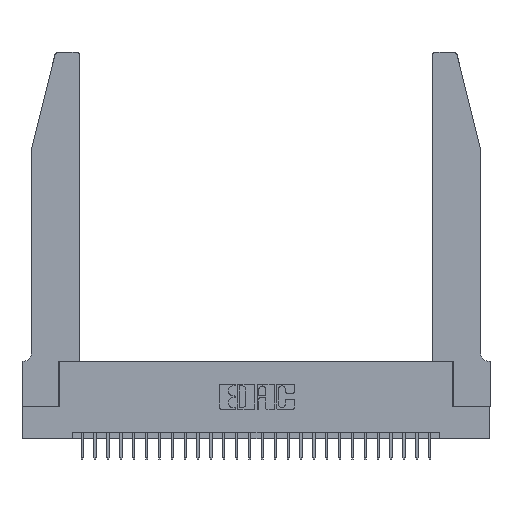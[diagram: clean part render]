
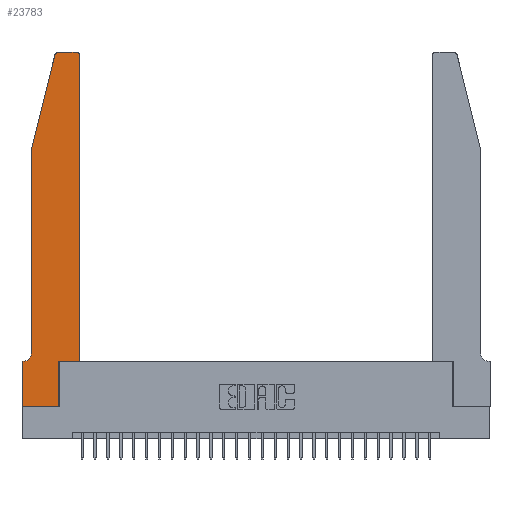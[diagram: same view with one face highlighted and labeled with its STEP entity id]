
A CAD part, top view. The second image highlights one B-rep face of the part: STEP entity #23783.
In plain terms, the highlighted planar face has unit normal (0, 0, 1).
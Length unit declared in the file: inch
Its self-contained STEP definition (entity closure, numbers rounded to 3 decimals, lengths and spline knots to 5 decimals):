
#187 = VERTEX_POINT ( 'NONE', #13765 ) ;
#409 = CARTESIAN_POINT ( 'NONE',  ( 0., 0., 0.37 ) ) ;
#474 = EDGE_LOOP ( 'NONE', ( #20091, #7254, #11517, #779, #2301, #14480, #12232, #7936, #6198, #28641, #19624, #24292 ) ) ;
#686 = AXIS2_PLACEMENT_3D ( 'NONE', #15063, #15173, #28624 ) ;
#774 = CARTESIAN_POINT ( 'NONE',  ( 0.2865, 0.35, 0.37 ) ) ;
#779 = ORIENTED_EDGE ( 'NONE', *, *, #18143, .T. ) ;
#855 = VERTEX_POINT ( 'NONE', #4358 ) ;
#983 = CARTESIAN_POINT ( 'NONE',  ( 0.0755, 2., 0.37 ) ) ;
#1223 = CARTESIAN_POINT ( 'NONE',  ( 0., 0.35, 0.37 ) ) ;
#1529 = AXIS2_PLACEMENT_3D ( 'NONE', #3961, #12609, #5810 ) ;
#2301 = ORIENTED_EDGE ( 'NONE', *, *, #15092, .T. ) ;
#3167 = VECTOR ( 'NONE', #26684, 39.37008 ) ;
#3686 = EDGE_CURVE ( 'NONE', #8865, #9156, #10705, .T. ) ;
#3943 = VECTOR ( 'NONE', #11604, 39.37008 ) ;
#3961 = CARTESIAN_POINT ( 'NONE',  ( 0.284, 2.72, 0.37 ) ) ;
#4107 = CARTESIAN_POINT ( 'NONE',  ( 0.4505, 0.35, 0.37 ) ) ;
#4358 = CARTESIAN_POINT ( 'NONE',  ( 0.4505, 2.72, 0.37 ) ) ;
#4560 = LINE ( 'NONE', #409, #3167 ) ;
#4834 = VECTOR ( 'NONE', #26246, 39.37008 ) ;
#5576 = DIRECTION ( 'NONE',  ( -0.239, -0.971, 0. ) ) ;
#5810 = DIRECTION ( 'NONE',  ( 1., 0., 0. ) ) ;
#6086 = DIRECTION ( 'NONE',  ( 1., 0., 0. ) ) ;
#6198 = ORIENTED_EDGE ( 'NONE', *, *, #3686, .T. ) ;
#6269 = LINE ( 'NONE', #23879, #4834 ) ;
#7254 = ORIENTED_EDGE ( 'NONE', *, *, #18571, .T. ) ;
#7544 = VERTEX_POINT ( 'NONE', #20810 ) ;
#7936 = ORIENTED_EDGE ( 'NONE', *, *, #14572, .T. ) ;
#7996 = PLANE ( 'NONE',  #16901 ) ;
#8092 = CIRCLE ( 'NONE', #1529, 0.03 ) ;
#8218 = DIRECTION ( 'NONE',  ( 0., 0., 1. ) ) ;
#8241 = CARTESIAN_POINT ( 'NONE',  ( 0.25487, 2.72718, 0.37 ) ) ;
#8254 = CARTESIAN_POINT ( 'NONE',  ( 0.284, 2.75, 0.37 ) ) ;
#8370 = CARTESIAN_POINT ( 'NONE',  ( 0.0755, 0.35, 0.37 ) ) ;
#8865 = VERTEX_POINT ( 'NONE', #10426 ) ;
#9140 = VECTOR ( 'NONE', #16576, 39.37008 ) ;
#9156 = VERTEX_POINT ( 'NONE', #10297 ) ;
#9300 = EDGE_CURVE ( 'NONE', #9156, #7544, #21344, .T. ) ;
#9340 = EDGE_CURVE ( 'NONE', #7544, #855, #20635, .T. ) ;
#9704 = DIRECTION ( 'NONE',  ( 0., 1., 0. ) ) ;
#9758 = DIRECTION ( 'NONE',  ( 1., 0., 0. ) ) ;
#9860 = VERTEX_POINT ( 'NONE', #14609 ) ;
#9937 = VECTOR ( 'NONE', #5576, 39.37008 ) ;
#10177 = DIRECTION ( 'NONE',  ( 0., 1., 0. ) ) ;
#10297 = CARTESIAN_POINT ( 'NONE',  ( 0.2865, 0.35, 0.37 ) ) ;
#10426 = CARTESIAN_POINT ( 'NONE',  ( 0.2865, 0., 0.37 ) ) ;
#10520 = DIRECTION ( 'NONE',  ( -1., 0., 0. ) ) ;
#10705 = LINE ( 'NONE', #774, #11374 ) ;
#10713 = VERTEX_POINT ( 'NONE', #22737 ) ;
#11374 = VECTOR ( 'NONE', #9704, 39.37008 ) ;
#11517 = ORIENTED_EDGE ( 'NONE', *, *, #16825, .T. ) ;
#11604 = DIRECTION ( 'NONE',  ( -1., 0., 0. ) ) ;
#12087 = VERTEX_POINT ( 'NONE', #12546 ) ;
#12232 = ORIENTED_EDGE ( 'NONE', *, *, #13995, .T. ) ;
#12546 = CARTESIAN_POINT ( 'NONE',  ( 0., 0.35, 0.37 ) ) ;
#12609 = DIRECTION ( 'NONE',  ( 0., 0., 1. ) ) ;
#13446 = FACE_OUTER_BOUND ( 'NONE', #474, .T. ) ;
#13765 = CARTESIAN_POINT ( 'NONE',  ( 0.4205, 2.75, 0.37 ) ) ;
#13995 = EDGE_CURVE ( 'NONE', #12087, #9860, #4560, .T. ) ;
#14399 = VERTEX_POINT ( 'NONE', #26976 ) ;
#14480 = ORIENTED_EDGE ( 'NONE', *, *, #16357, .T. ) ;
#14572 = EDGE_CURVE ( 'NONE', #9860, #8865, #6269, .T. ) ;
#14609 = CARTESIAN_POINT ( 'NONE',  ( 0., 0., 0.37 ) ) ;
#14823 = EDGE_CURVE ( 'NONE', #855, #187, #21125, .T. ) ;
#14831 = LINE ( 'NONE', #8370, #26615 ) ;
#14850 = CARTESIAN_POINT ( 'NONE',  ( 0.2605, 2.75, 0.37 ) ) ;
#15063 = CARTESIAN_POINT ( 'NONE',  ( 0.0055, 0.42, 0.37 ) ) ;
#15092 = EDGE_CURVE ( 'NONE', #17347, #14399, #21803, .T. ) ;
#15173 = DIRECTION ( 'NONE',  ( 0., 0., -1. ) ) ;
#15710 = LINE ( 'NONE', #14850, #3943 ) ;
#16357 = EDGE_CURVE ( 'NONE', #14399, #12087, #14831, .T. ) ;
#16576 = DIRECTION ( 'NONE',  ( 0., -1., 0. ) ) ;
#16825 = EDGE_CURVE ( 'NONE', #28004, #10713, #20994, .T. ) ;
#16901 = AXIS2_PLACEMENT_3D ( 'NONE', #1223, #18838, #9758 ) ;
#16982 = CARTESIAN_POINT ( 'NONE',  ( 0.4505, 0.35, 0.37 ) ) ;
#17347 = VERTEX_POINT ( 'NONE', #21845 ) ;
#17777 = VERTEX_POINT ( 'NONE', #8254 ) ;
#18143 = EDGE_CURVE ( 'NONE', #10713, #17347, #27536, .T. ) ;
#18571 = EDGE_CURVE ( 'NONE', #17777, #28004, #8092, .T. ) ;
#18838 = DIRECTION ( 'NONE',  ( 0., 0., 1. ) ) ;
#19071 = EDGE_CURVE ( 'NONE', #187, #17777, #15710, .T. ) ;
#19091 = DIRECTION ( 'NONE',  ( 1., 0., 0. ) ) ;
#19535 = CARTESIAN_POINT ( 'NONE',  ( 0.4205, 2.72, 0.37 ) ) ;
#19624 = ORIENTED_EDGE ( 'NONE', *, *, #9340, .T. ) ;
#20091 = ORIENTED_EDGE ( 'NONE', *, *, #19071, .T. ) ;
#20635 = LINE ( 'NONE', #4107, #28337 ) ;
#20810 = CARTESIAN_POINT ( 'NONE',  ( 0.4505, 0.35, 0.37 ) ) ;
#20994 = LINE ( 'NONE', #27478, #9937 ) ;
#21125 = CIRCLE ( 'NONE', #27046, 0.03 ) ;
#21344 = LINE ( 'NONE', #16982, #22705 ) ;
#21803 = CIRCLE ( 'NONE', #686, 0.07 ) ;
#21845 = CARTESIAN_POINT ( 'NONE',  ( 0.0755, 0.42, 0.37 ) ) ;
#22705 = VECTOR ( 'NONE', #19091, 39.37008 ) ;
#22737 = CARTESIAN_POINT ( 'NONE',  ( 0.0755, 2., 0.37 ) ) ;
#23783 = ADVANCED_FACE ( 'NONE', ( #13446 ), #7996, .T. ) ;
#23879 = CARTESIAN_POINT ( 'NONE',  ( 0., 0., 0.37 ) ) ;
#24292 = ORIENTED_EDGE ( 'NONE', *, *, #14823, .T. ) ;
#26246 = DIRECTION ( 'NONE',  ( 1., 0., 0. ) ) ;
#26615 = VECTOR ( 'NONE', #10520, 39.37008 ) ;
#26684 = DIRECTION ( 'NONE',  ( 0., -1., 0. ) ) ;
#26976 = CARTESIAN_POINT ( 'NONE',  ( 0.0055, 0.35, 0.37 ) ) ;
#27046 = AXIS2_PLACEMENT_3D ( 'NONE', #19535, #8218, #6086 ) ;
#27478 = CARTESIAN_POINT ( 'NONE',  ( 0.0755, 2., 0.37 ) ) ;
#27536 = LINE ( 'NONE', #983, #9140 ) ;
#28004 = VERTEX_POINT ( 'NONE', #8241 ) ;
#28337 = VECTOR ( 'NONE', #10177, 39.37008 ) ;
#28624 = DIRECTION ( 'NONE',  ( -1., 0., 0. ) ) ;
#28641 = ORIENTED_EDGE ( 'NONE', *, *, #9300, .T. ) ;
